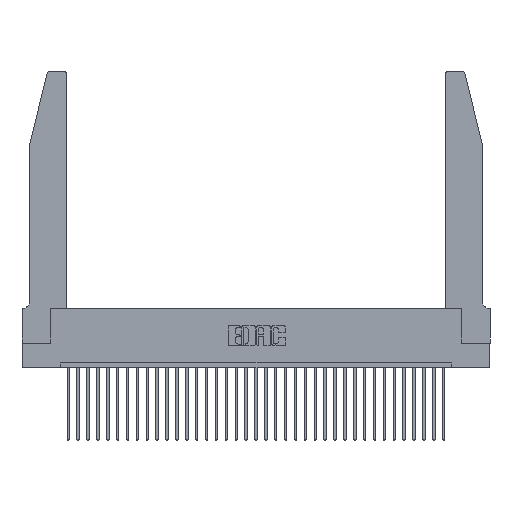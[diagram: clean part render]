
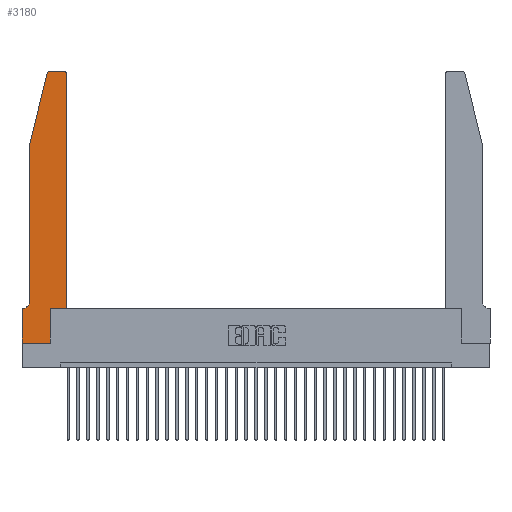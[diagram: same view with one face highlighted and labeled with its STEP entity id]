
A CAD part, top view. The second image highlights one B-rep face of the part: STEP entity #3180.
In plain terms, the highlighted planar face has unit normal (0, 0, 1).
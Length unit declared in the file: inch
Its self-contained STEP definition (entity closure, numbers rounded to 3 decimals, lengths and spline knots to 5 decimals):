
#360 = VERTEX_POINT ( 'NONE', #21402 ) ;
#710 = VERTEX_POINT ( 'NONE', #6821 ) ;
#1846 = DIRECTION ( 'NONE',  ( -0.239, -0.971, 0. ) ) ;
#1940 = AXIS2_PLACEMENT_3D ( 'NONE', #2701, #24900, #32853 ) ;
#2287 = VECTOR ( 'NONE', #10397, 39.37008 ) ;
#2701 = CARTESIAN_POINT ( 'NONE',  ( 0.0055, 0.42, 0.37 ) ) ;
#2966 = VERTEX_POINT ( 'NONE', #26050 ) ;
#3180 = ADVANCED_FACE ( 'NONE', ( #5234 ), #31664, .T. ) ;
#3841 = DIRECTION ( 'NONE',  ( -1., 0., 0. ) ) ;
#4288 = VERTEX_POINT ( 'NONE', #24497 ) ;
#4506 = CARTESIAN_POINT ( 'NONE',  ( 0., 0., 0.37 ) ) ;
#4766 = DIRECTION ( 'NONE',  ( 1., 0., 0. ) ) ;
#5111 = VECTOR ( 'NONE', #1846, 39.37008 ) ;
#5234 = FACE_OUTER_BOUND ( 'NONE', #6663, .T. ) ;
#5310 = LINE ( 'NONE', #10002, #30292 ) ;
#6326 = EDGE_CURVE ( 'NONE', #29021, #360, #10837, .T. ) ;
#6663 = EDGE_LOOP ( 'NONE', ( #6750, #34311, #25957, #23036, #11224, #22553, #34326, #17129, #27540, #23855, #18203, #16688 ) ) ;
#6750 = ORIENTED_EDGE ( 'NONE', *, *, #20550, .T. ) ;
#6819 = VECTOR ( 'NONE', #29324, 39.37008 ) ;
#6821 = CARTESIAN_POINT ( 'NONE',  ( 0.0055, 0.35, 0.37 ) ) ;
#9130 = CARTESIAN_POINT ( 'NONE',  ( 0., 0., 0.37 ) ) ;
#9365 = CARTESIAN_POINT ( 'NONE',  ( 0.284, 2.72, 0.37 ) ) ;
#9974 = CARTESIAN_POINT ( 'NONE',  ( 0.0755, 2., 0.37 ) ) ;
#10002 = CARTESIAN_POINT ( 'NONE',  ( 0.0755, 2., 0.37 ) ) ;
#10397 = DIRECTION ( 'NONE',  ( 0., 1., 0. ) ) ;
#10402 = EDGE_CURVE ( 'NONE', #28942, #14636, #5310, .T. ) ;
#10577 = DIRECTION ( 'NONE',  ( -1., 0., 0. ) ) ;
#10837 = LINE ( 'NONE', #4506, #31262 ) ;
#11224 = ORIENTED_EDGE ( 'NONE', *, *, #14209, .T. ) ;
#11340 = CARTESIAN_POINT ( 'NONE',  ( 0.4205, 2.72, 0.37 ) ) ;
#11343 = EDGE_CURVE ( 'NONE', #710, #22531, #34028, .T. ) ;
#11499 = AXIS2_PLACEMENT_3D ( 'NONE', #9365, #32778, #19392 ) ;
#11560 = DIRECTION ( 'NONE',  ( 1., 0., 0. ) ) ;
#13211 = DIRECTION ( 'NONE',  ( 1., 0., 0. ) ) ;
#13471 = VECTOR ( 'NONE', #22678, 39.37008 ) ;
#14045 = CARTESIAN_POINT ( 'NONE',  ( 0.284, 2.75, 0.37 ) ) ;
#14209 = EDGE_CURVE ( 'NONE', #14636, #710, #17689, .T. ) ;
#14636 = VERTEX_POINT ( 'NONE', #27422 ) ;
#14721 = CARTESIAN_POINT ( 'NONE',  ( 0., 0.35, 0.37 ) ) ;
#15047 = VERTEX_POINT ( 'NONE', #14045 ) ;
#15189 = LINE ( 'NONE', #23604, #24305 ) ;
#16203 = EDGE_CURVE ( 'NONE', #23750, #28758, #31485, .T. ) ;
#16296 = EDGE_CURVE ( 'NONE', #19927, #23750, #19833, .T. ) ;
#16688 = ORIENTED_EDGE ( 'NONE', *, *, #16203, .T. ) ;
#17129 = ORIENTED_EDGE ( 'NONE', *, *, #6326, .T. ) ;
#17689 = CIRCLE ( 'NONE', #1940, 0.07 ) ;
#18203 = ORIENTED_EDGE ( 'NONE', *, *, #16296, .T. ) ;
#18222 = LINE ( 'NONE', #34473, #25721 ) ;
#18295 = DIRECTION ( 'NONE',  ( 0., -1., 0. ) ) ;
#19328 = CARTESIAN_POINT ( 'NONE',  ( 0.0755, 0.35, 0.37 ) ) ;
#19392 = DIRECTION ( 'NONE',  ( 1., 0., 0. ) ) ;
#19833 = LINE ( 'NONE', #26115, #2287 ) ;
#19927 = VERTEX_POINT ( 'NONE', #29226 ) ;
#20550 = EDGE_CURVE ( 'NONE', #28758, #15047, #18222, .T. ) ;
#20640 = CARTESIAN_POINT ( 'NONE',  ( 0., 0.35, 0.37 ) ) ;
#21402 = CARTESIAN_POINT ( 'NONE',  ( 0.2865, 0., 0.37 ) ) ;
#21649 = CARTESIAN_POINT ( 'NONE',  ( 0.2865, 0.35, 0.37 ) ) ;
#21766 = LINE ( 'NONE', #9974, #5111 ) ;
#21860 = CARTESIAN_POINT ( 'NONE',  ( 0.4205, 2.75, 0.37 ) ) ;
#22457 = CARTESIAN_POINT ( 'NONE',  ( 0.0755, 2., 0.37 ) ) ;
#22531 = VERTEX_POINT ( 'NONE', #14721 ) ;
#22553 = ORIENTED_EDGE ( 'NONE', *, *, #11343, .T. ) ;
#22678 = DIRECTION ( 'NONE',  ( 0., -1., 0. ) ) ;
#23036 = ORIENTED_EDGE ( 'NONE', *, *, #10402, .T. ) ;
#23604 = CARTESIAN_POINT ( 'NONE',  ( 0.4505, 0.35, 0.37 ) ) ;
#23750 = VERTEX_POINT ( 'NONE', #30986 ) ;
#23855 = ORIENTED_EDGE ( 'NONE', *, *, #26404, .T. ) ;
#24305 = VECTOR ( 'NONE', #13211, 39.37008 ) ;
#24497 = CARTESIAN_POINT ( 'NONE',  ( 0.25487, 2.72718, 0.37 ) ) ;
#24688 = LINE ( 'NONE', #21649, #6819 ) ;
#24900 = DIRECTION ( 'NONE',  ( 0., 0., -1. ) ) ;
#25721 = VECTOR ( 'NONE', #10577, 39.37008 ) ;
#25957 = ORIENTED_EDGE ( 'NONE', *, *, #34462, .T. ) ;
#26050 = CARTESIAN_POINT ( 'NONE',  ( 0.2865, 0.35, 0.37 ) ) ;
#26115 = CARTESIAN_POINT ( 'NONE',  ( 0.4505, 0.35, 0.37 ) ) ;
#26404 = EDGE_CURVE ( 'NONE', #2966, #19927, #15189, .T. ) ;
#26610 = EDGE_CURVE ( 'NONE', #22531, #29021, #28049, .T. ) ;
#26861 = VECTOR ( 'NONE', #3841, 39.37008 ) ;
#26888 = AXIS2_PLACEMENT_3D ( 'NONE', #20640, #28604, #4766 ) ;
#27422 = CARTESIAN_POINT ( 'NONE',  ( 0.0755, 0.42, 0.37 ) ) ;
#27491 = CIRCLE ( 'NONE', #11499, 0.03 ) ;
#27505 = DIRECTION ( 'NONE',  ( 0., 0., 1. ) ) ;
#27540 = ORIENTED_EDGE ( 'NONE', *, *, #34057, .T. ) ;
#27598 = AXIS2_PLACEMENT_3D ( 'NONE', #11340, #27505, #27637 ) ;
#27637 = DIRECTION ( 'NONE',  ( 1., 0., 0. ) ) ;
#27866 = EDGE_CURVE ( 'NONE', #15047, #4288, #27491, .T. ) ;
#28005 = CARTESIAN_POINT ( 'NONE',  ( 0., 0., 0.37 ) ) ;
#28049 = LINE ( 'NONE', #9130, #13471 ) ;
#28604 = DIRECTION ( 'NONE',  ( 0., 0., 1. ) ) ;
#28758 = VERTEX_POINT ( 'NONE', #21860 ) ;
#28942 = VERTEX_POINT ( 'NONE', #22457 ) ;
#29021 = VERTEX_POINT ( 'NONE', #28005 ) ;
#29226 = CARTESIAN_POINT ( 'NONE',  ( 0.4505, 0.35, 0.37 ) ) ;
#29324 = DIRECTION ( 'NONE',  ( 0., 1., 0. ) ) ;
#30292 = VECTOR ( 'NONE', #18295, 39.37008 ) ;
#30986 = CARTESIAN_POINT ( 'NONE',  ( 0.4505, 2.72, 0.37 ) ) ;
#31262 = VECTOR ( 'NONE', #11560, 39.37008 ) ;
#31485 = CIRCLE ( 'NONE', #27598, 0.03 ) ;
#31664 = PLANE ( 'NONE',  #26888 ) ;
#32778 = DIRECTION ( 'NONE',  ( 0., 0., 1. ) ) ;
#32853 = DIRECTION ( 'NONE',  ( -1., 0., 0. ) ) ;
#34028 = LINE ( 'NONE', #19328, #26861 ) ;
#34057 = EDGE_CURVE ( 'NONE', #360, #2966, #24688, .T. ) ;
#34311 = ORIENTED_EDGE ( 'NONE', *, *, #27866, .T. ) ;
#34326 = ORIENTED_EDGE ( 'NONE', *, *, #26610, .T. ) ;
#34462 = EDGE_CURVE ( 'NONE', #4288, #28942, #21766, .T. ) ;
#34473 = CARTESIAN_POINT ( 'NONE',  ( 0.2605, 2.75, 0.37 ) ) ;
